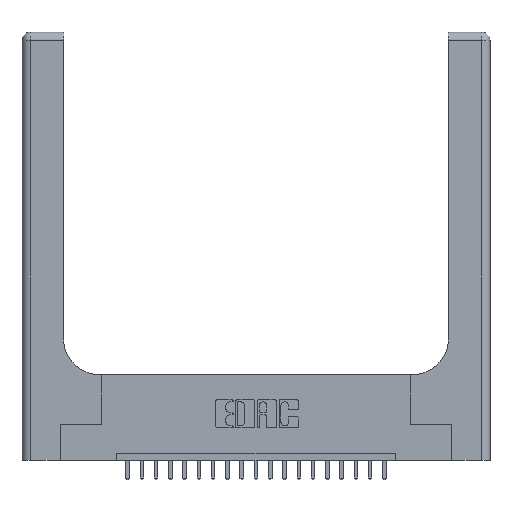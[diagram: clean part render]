
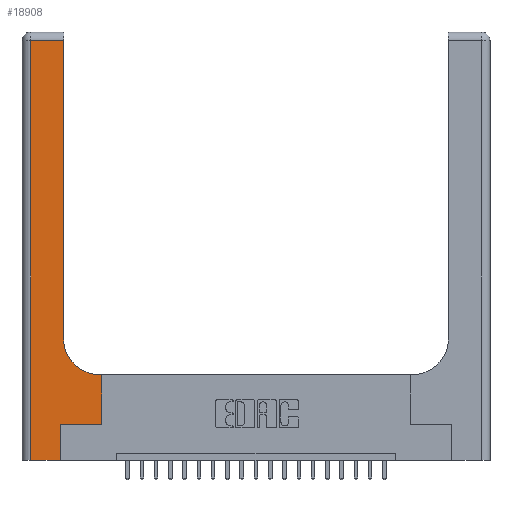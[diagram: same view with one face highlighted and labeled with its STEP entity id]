
A CAD part, top view. The second image highlights one B-rep face of the part: STEP entity #18908.
In plain terms, the highlighted planar face has unit normal (0, 0, 1).
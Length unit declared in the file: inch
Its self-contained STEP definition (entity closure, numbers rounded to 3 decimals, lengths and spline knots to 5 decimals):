
#493 = EDGE_LOOP ( 'NONE', ( #4480, #1695, #7488, #13228, #14793, #15367, #21960, #8690, #12970 ) ) ;
#830 = LINE ( 'NONE', #21510, #8734 ) ;
#1239 = CARTESIAN_POINT ( 'NONE',  ( 0.5585, 0.25, 0.37 ) ) ;
#1339 = VECTOR ( 'NONE', #2638, 39.37008 ) ;
#1695 = ORIENTED_EDGE ( 'NONE', *, *, #8958, .T. ) ;
#2139 = CARTESIAN_POINT ( 'NONE',  ( 0.5415, 0.85, 0.37 ) ) ;
#2493 = VECTOR ( 'NONE', #7986, 39.37008 ) ;
#2518 = LINE ( 'NONE', #1239, #12615 ) ;
#2583 = VERTEX_POINT ( 'NONE', #19412 ) ;
#2638 = DIRECTION ( 'NONE',  ( 1., 0., 0. ) ) ;
#3304 = EDGE_CURVE ( 'NONE', #2583, #3725, #5471, .T. ) ;
#3327 = VERTEX_POINT ( 'NONE', #13225 ) ;
#3725 = VERTEX_POINT ( 'NONE', #21374 ) ;
#3731 = CARTESIAN_POINT ( 'NONE',  ( 0.2915, 0.85, 0.37 ) ) ;
#4311 = DIRECTION ( 'NONE',  ( 0., -1., 0. ) ) ;
#4442 = VERTEX_POINT ( 'NONE', #11371 ) ;
#4480 = ORIENTED_EDGE ( 'NONE', *, *, #9156, .T. ) ;
#5471 = LINE ( 'NONE', #14923, #2493 ) ;
#5639 = DIRECTION ( 'NONE',  ( 1., 0., 0. ) ) ;
#6266 = VECTOR ( 'NONE', #17051, 39.37008 ) ;
#7228 = DIRECTION ( 'NONE',  ( 0., 1., 0. ) ) ;
#7325 = VECTOR ( 'NONE', #21450, 39.37008 ) ;
#7370 = AXIS2_PLACEMENT_3D ( 'NONE', #11419, #20869, #21291 ) ;
#7488 = ORIENTED_EDGE ( 'NONE', *, *, #21064, .T. ) ;
#7561 = CIRCLE ( 'NONE', #21843, 0.25 ) ;
#7589 = DIRECTION ( 'NONE',  ( -1., 0., 0. ) ) ;
#7986 = DIRECTION ( 'NONE',  ( -1., 0., 0. ) ) ;
#8074 = EDGE_CURVE ( 'NONE', #3327, #2583, #2518, .T. ) ;
#8227 = VERTEX_POINT ( 'NONE', #13564 ) ;
#8690 = ORIENTED_EDGE ( 'NONE', *, *, #3304, .T. ) ;
#8722 = VECTOR ( 'NONE', #7589, 39.37008 ) ;
#8734 = VECTOR ( 'NONE', #4311, 39.37008 ) ;
#8958 = EDGE_CURVE ( 'NONE', #8227, #4442, #21523, .T. ) ;
#9156 = EDGE_CURVE ( 'NONE', #15772, #8227, #10948, .T. ) ;
#9675 = CARTESIAN_POINT ( 'NONE',  ( 0.269, 0.25, 0.37 ) ) ;
#9701 = EDGE_CURVE ( 'NONE', #15860, #3327, #22335, .T. ) ;
#10941 = CARTESIAN_POINT ( 'NONE',  ( 0.269, 0., 0.37 ) ) ;
#10948 = LINE ( 'NONE', #15206, #6266 ) ;
#11371 = CARTESIAN_POINT ( 'NONE',  ( 0.06, 2.94, 0.37 ) ) ;
#11419 = CARTESIAN_POINT ( 'NONE',  ( 0., 3., 0.37 ) ) ;
#12615 = VECTOR ( 'NONE', #7228, 39.37008 ) ;
#12714 = CARTESIAN_POINT ( 'NONE',  ( 0., 0., 0.37 ) ) ;
#12777 = CARTESIAN_POINT ( 'NONE',  ( 0.06, 0., 0.37 ) ) ;
#12970 = ORIENTED_EDGE ( 'NONE', *, *, #17546, .T. ) ;
#13225 = CARTESIAN_POINT ( 'NONE',  ( 0.5585, 0.25, 0.37 ) ) ;
#13228 = ORIENTED_EDGE ( 'NONE', *, *, #16818, .T. ) ;
#13564 = CARTESIAN_POINT ( 'NONE',  ( 0.2915, 2.94, 0.37 ) ) ;
#13805 = CARTESIAN_POINT ( 'NONE',  ( 0.269, 0., 0.37 ) ) ;
#13851 = FACE_OUTER_BOUND ( 'NONE', #493, .T. ) ;
#14448 = PLANE ( 'NONE',  #7370 ) ;
#14793 = ORIENTED_EDGE ( 'NONE', *, *, #22456, .T. ) ;
#14923 = CARTESIAN_POINT ( 'NONE',  ( 0.2915, 0.6, 0.37 ) ) ;
#15206 = CARTESIAN_POINT ( 'NONE',  ( 0.2915, 3., 0.37 ) ) ;
#15367 = ORIENTED_EDGE ( 'NONE', *, *, #9701, .T. ) ;
#15772 = VERTEX_POINT ( 'NONE', #3731 ) ;
#15860 = VERTEX_POINT ( 'NONE', #9675 ) ;
#16074 = DIRECTION ( 'NONE',  ( 0., 0., -1. ) ) ;
#16601 = LINE ( 'NONE', #12714, #7325 ) ;
#16818 = EDGE_CURVE ( 'NONE', #19318, #21674, #16601, .T. ) ;
#16860 = CARTESIAN_POINT ( 'NONE',  ( 0.269, 0.25, 0.37 ) ) ;
#17051 = DIRECTION ( 'NONE',  ( 0., 1., 0. ) ) ;
#17385 = LINE ( 'NONE', #13805, #18749 ) ;
#17546 = EDGE_CURVE ( 'NONE', #3725, #15772, #7561, .T. ) ;
#18749 = VECTOR ( 'NONE', #22338, 39.37008 ) ;
#18908 = ADVANCED_FACE ( 'NONE', ( #13851 ), #14448, .F. ) ;
#19318 = VERTEX_POINT ( 'NONE', #12777 ) ;
#19412 = CARTESIAN_POINT ( 'NONE',  ( 0.5585, 0.6, 0.37 ) ) ;
#19878 = CARTESIAN_POINT ( 'NONE',  ( 0., 2.94, 0.37 ) ) ;
#20869 = DIRECTION ( 'NONE',  ( 0., 0., -1. ) ) ;
#21064 = EDGE_CURVE ( 'NONE', #4442, #19318, #830, .T. ) ;
#21291 = DIRECTION ( 'NONE',  ( -1., 0., 0. ) ) ;
#21374 = CARTESIAN_POINT ( 'NONE',  ( 0.5415, 0.6, 0.37 ) ) ;
#21450 = DIRECTION ( 'NONE',  ( 1., 0., 0. ) ) ;
#21510 = CARTESIAN_POINT ( 'NONE',  ( 0.06, 3., 0.37 ) ) ;
#21523 = LINE ( 'NONE', #19878, #8722 ) ;
#21674 = VERTEX_POINT ( 'NONE', #10941 ) ;
#21843 = AXIS2_PLACEMENT_3D ( 'NONE', #2139, #16074, #5639 ) ;
#21960 = ORIENTED_EDGE ( 'NONE', *, *, #8074, .T. ) ;
#22335 = LINE ( 'NONE', #16860, #1339 ) ;
#22338 = DIRECTION ( 'NONE',  ( 0., 1., 0. ) ) ;
#22456 = EDGE_CURVE ( 'NONE', #21674, #15860, #17385, .T. ) ;
